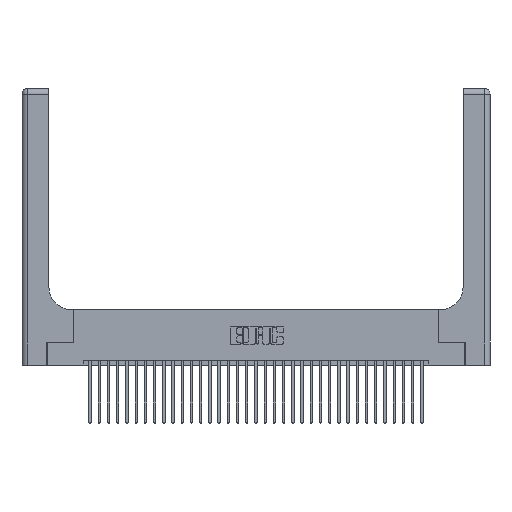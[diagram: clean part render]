
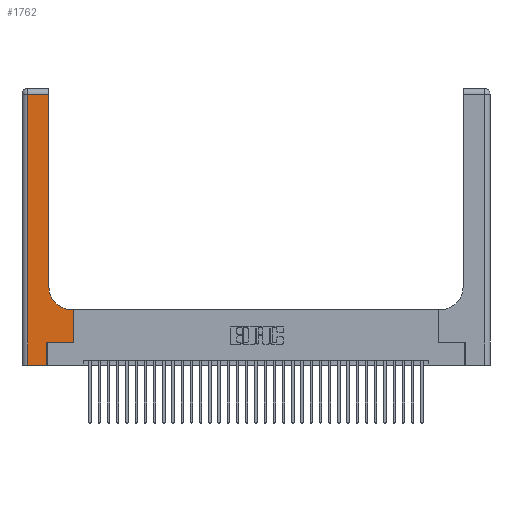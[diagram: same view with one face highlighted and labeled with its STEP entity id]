
A CAD part, top view. The second image highlights one B-rep face of the part: STEP entity #1762.
In plain terms, the highlighted planar face has unit normal (0, 0, 1).
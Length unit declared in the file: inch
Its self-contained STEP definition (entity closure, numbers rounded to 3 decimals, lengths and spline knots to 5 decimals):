
#72 = EDGE_CURVE ( 'NONE', #13672, #6011, #20841, .T. ) ;
#331 = ORIENTED_EDGE ( 'NONE', *, *, #20529, .T. ) ;
#495 = DIRECTION ( 'NONE',  ( -1., 0., 0. ) ) ;
#635 = EDGE_CURVE ( 'NONE', #31135, #778, #7573, .T. ) ;
#778 = VERTEX_POINT ( 'NONE', #27070 ) ;
#1083 = VERTEX_POINT ( 'NONE', #20612 ) ;
#1208 = DIRECTION ( 'NONE',  ( 0., -1., 0. ) ) ;
#1647 = VECTOR ( 'NONE', #22394, 39.37008 ) ;
#1762 = ADVANCED_FACE ( 'NONE', ( #28676 ), #21497, .F. ) ;
#2222 = CIRCLE ( 'NONE', #4665, 0.25 ) ;
#2254 = EDGE_LOOP ( 'NONE', ( #10921, #22527, #34111, #11122, #6238, #27664, #331, #3300, #14723 ) ) ;
#2567 = EDGE_CURVE ( 'NONE', #29169, #27305, #15115, .T. ) ;
#3133 = DIRECTION ( 'NONE',  ( 0., 0., -1. ) ) ;
#3209 = CARTESIAN_POINT ( 'NONE',  ( 0., 2.94, 0.37 ) ) ;
#3300 = ORIENTED_EDGE ( 'NONE', *, *, #635, .T. ) ;
#3775 = CARTESIAN_POINT ( 'NONE',  ( 0.269, 0., 0.37 ) ) ;
#3833 = CARTESIAN_POINT ( 'NONE',  ( 0.06, 3., 0.37 ) ) ;
#4665 = AXIS2_PLACEMENT_3D ( 'NONE', #31561, #34244, #12528 ) ;
#4721 = LINE ( 'NONE', #8266, #15720 ) ;
#4773 = CARTESIAN_POINT ( 'NONE',  ( 0.5585, 0.25, 0.37 ) ) ;
#6011 = VERTEX_POINT ( 'NONE', #34221 ) ;
#6149 = DIRECTION ( 'NONE',  ( -1., 0., 0. ) ) ;
#6165 = EDGE_CURVE ( 'NONE', #27305, #22384, #7231, .T. ) ;
#6238 = ORIENTED_EDGE ( 'NONE', *, *, #23983, .T. ) ;
#6842 = CARTESIAN_POINT ( 'NONE',  ( 0.2915, 2.94, 0.37 ) ) ;
#7213 = VECTOR ( 'NONE', #28748, 39.37008 ) ;
#7231 = LINE ( 'NONE', #3833, #18259 ) ;
#7573 = LINE ( 'NONE', #30775, #1647 ) ;
#8037 = CARTESIAN_POINT ( 'NONE',  ( 0.269, 0.25, 0.37 ) ) ;
#8266 = CARTESIAN_POINT ( 'NONE',  ( 0.2915, 3., 0.37 ) ) ;
#8392 = CARTESIAN_POINT ( 'NONE',  ( 0., 3., 0.37 ) ) ;
#10115 = CARTESIAN_POINT ( 'NONE',  ( 0., 0., 0.37 ) ) ;
#10921 = ORIENTED_EDGE ( 'NONE', *, *, #34659, .T. ) ;
#11122 = ORIENTED_EDGE ( 'NONE', *, *, #23130, .T. ) ;
#12150 = CARTESIAN_POINT ( 'NONE',  ( 0.06, 0., 0.37 ) ) ;
#12528 = DIRECTION ( 'NONE',  ( 1., 0., 0. ) ) ;
#13526 = DIRECTION ( 'NONE',  ( 1., 0., 0. ) ) ;
#13672 = VERTEX_POINT ( 'NONE', #33372 ) ;
#14407 = LINE ( 'NONE', #4773, #7213 ) ;
#14723 = ORIENTED_EDGE ( 'NONE', *, *, #25520, .T. ) ;
#14834 = CARTESIAN_POINT ( 'NONE',  ( 0.2915, 0.85, 0.37 ) ) ;
#15115 = LINE ( 'NONE', #3209, #27735 ) ;
#15720 = VECTOR ( 'NONE', #24599, 39.37008 ) ;
#16303 = LINE ( 'NONE', #3775, #31078 ) ;
#16795 = CARTESIAN_POINT ( 'NONE',  ( 0.06, 2.94, 0.37 ) ) ;
#17399 = DIRECTION ( 'NONE',  ( 0., 1., 0. ) ) ;
#18259 = VECTOR ( 'NONE', #1208, 39.37008 ) ;
#20232 = CARTESIAN_POINT ( 'NONE',  ( 0.5585, 0.6, 0.37 ) ) ;
#20529 = EDGE_CURVE ( 'NONE', #6011, #31135, #14407, .T. ) ;
#20558 = LINE ( 'NONE', #10115, #28095 ) ;
#20612 = CARTESIAN_POINT ( 'NONE',  ( 0.269, 0., 0.37 ) ) ;
#20841 = LINE ( 'NONE', #8037, #32208 ) ;
#21497 = PLANE ( 'NONE',  #29456 ) ;
#22384 = VERTEX_POINT ( 'NONE', #12150 ) ;
#22394 = DIRECTION ( 'NONE',  ( -1., 0., 0. ) ) ;
#22527 = ORIENTED_EDGE ( 'NONE', *, *, #2567, .T. ) ;
#23130 = EDGE_CURVE ( 'NONE', #22384, #1083, #20558, .T. ) ;
#23625 = DIRECTION ( 'NONE',  ( 1., 0., 0. ) ) ;
#23983 = EDGE_CURVE ( 'NONE', #1083, #13672, #16303, .T. ) ;
#24599 = DIRECTION ( 'NONE',  ( 0., 1., 0. ) ) ;
#25520 = EDGE_CURVE ( 'NONE', #778, #30501, #2222, .T. ) ;
#27070 = CARTESIAN_POINT ( 'NONE',  ( 0.5415, 0.6, 0.37 ) ) ;
#27305 = VERTEX_POINT ( 'NONE', #16795 ) ;
#27664 = ORIENTED_EDGE ( 'NONE', *, *, #72, .T. ) ;
#27735 = VECTOR ( 'NONE', #6149, 39.37008 ) ;
#28095 = VECTOR ( 'NONE', #23625, 39.37008 ) ;
#28676 = FACE_OUTER_BOUND ( 'NONE', #2254, .T. ) ;
#28748 = DIRECTION ( 'NONE',  ( 0., 1., 0. ) ) ;
#29169 = VERTEX_POINT ( 'NONE', #6842 ) ;
#29456 = AXIS2_PLACEMENT_3D ( 'NONE', #8392, #3133, #495 ) ;
#30501 = VERTEX_POINT ( 'NONE', #14834 ) ;
#30775 = CARTESIAN_POINT ( 'NONE',  ( 0.2915, 0.6, 0.37 ) ) ;
#31078 = VECTOR ( 'NONE', #17399, 39.37008 ) ;
#31135 = VERTEX_POINT ( 'NONE', #20232 ) ;
#31561 = CARTESIAN_POINT ( 'NONE',  ( 0.5415, 0.85, 0.37 ) ) ;
#32208 = VECTOR ( 'NONE', #13526, 39.37008 ) ;
#33372 = CARTESIAN_POINT ( 'NONE',  ( 0.269, 0.25, 0.37 ) ) ;
#34111 = ORIENTED_EDGE ( 'NONE', *, *, #6165, .T. ) ;
#34221 = CARTESIAN_POINT ( 'NONE',  ( 0.5585, 0.25, 0.37 ) ) ;
#34244 = DIRECTION ( 'NONE',  ( 0., 0., -1. ) ) ;
#34659 = EDGE_CURVE ( 'NONE', #30501, #29169, #4721, .T. ) ;
